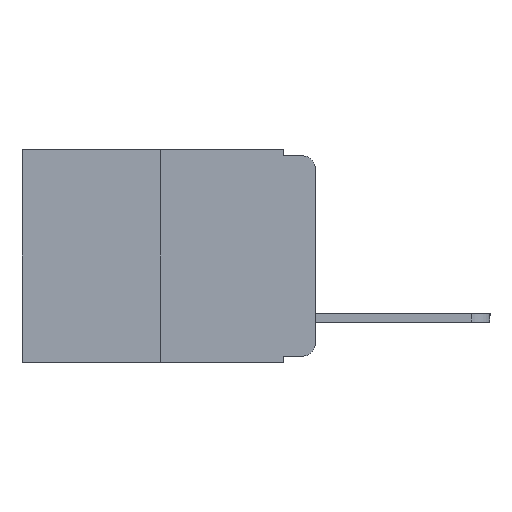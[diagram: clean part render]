
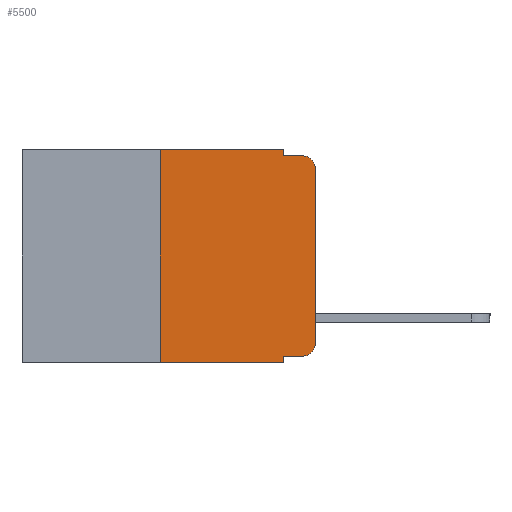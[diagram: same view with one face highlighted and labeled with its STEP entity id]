
A CAD part, left-side view. The second image highlights one B-rep face of the part: STEP entity #5500.
In plain terms, the highlighted planar face has unit normal (-1, 0, 0).
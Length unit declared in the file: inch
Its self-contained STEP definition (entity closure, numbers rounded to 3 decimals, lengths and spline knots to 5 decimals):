
#333 = VERTEX_POINT ( 'NONE', #11240 ) ;
#370 = LINE ( 'NONE', #1145, #9718 ) ;
#388 = CIRCLE ( 'NONE', #5598, 0.02 ) ;
#451 = VERTEX_POINT ( 'NONE', #4554 ) ;
#977 = DIRECTION ( 'NONE',  ( 0., -1., 0. ) ) ;
#1043 = DIRECTION ( 'NONE',  ( 0., -1., 0. ) ) ;
#1145 = CARTESIAN_POINT ( 'NONE',  ( 0., 0.473, 0. ) ) ;
#1429 = VERTEX_POINT ( 'NONE', #10984 ) ;
#1430 = VERTEX_POINT ( 'NONE', #10997 ) ;
#1515 = EDGE_CURVE ( 'NONE', #451, #1429, #10288, .T. ) ;
#1613 = CARTESIAN_POINT ( 'NONE',  ( 0., 0., 0. ) ) ;
#1649 = VERTEX_POINT ( 'NONE', #6279 ) ;
#1702 = DIRECTION ( 'NONE',  ( -1., 0., 0. ) ) ;
#1745 = CARTESIAN_POINT ( 'NONE',  ( 0., 0.051, -0.343 ) ) ;
#1945 = LINE ( 'NONE', #4502, #10922 ) ;
#2081 = VERTEX_POINT ( 'NONE', #5984 ) ;
#2215 = VECTOR ( 'NONE', #11425, 39.37008 ) ;
#2300 = CARTESIAN_POINT ( 'NONE',  ( 0., 0.473, -0.343 ) ) ;
#2356 = ORIENTED_EDGE ( 'NONE', *, *, #10770, .T. ) ;
#2634 = LINE ( 'NONE', #7529, #9096 ) ;
#2791 = ORIENTED_EDGE ( 'NONE', *, *, #8712, .F. ) ;
#3426 = DIRECTION ( 'NONE',  ( 0., 0., 1. ) ) ;
#3429 = VERTEX_POINT ( 'NONE', #6857 ) ;
#3449 = LINE ( 'NONE', #7114, #5597 ) ;
#4209 = EDGE_LOOP ( 'NONE', ( #5742, #10328, #10606, #4535, #4773, #2791, #10747, #4414, #11284, #2356 ) ) ;
#4414 = ORIENTED_EDGE ( 'NONE', *, *, #9178, .F. ) ;
#4502 = CARTESIAN_POINT ( 'NONE',  ( 0., 0.051, -0.01 ) ) ;
#4535 = ORIENTED_EDGE ( 'NONE', *, *, #8375, .F. ) ;
#4554 = CARTESIAN_POINT ( 'NONE',  ( 0., 0., -0.03 ) ) ;
#4773 = ORIENTED_EDGE ( 'NONE', *, *, #5081, .F. ) ;
#5035 = VERTEX_POINT ( 'NONE', #1745 ) ;
#5081 = EDGE_CURVE ( 'NONE', #3429, #333, #370, .T. ) ;
#5314 = LINE ( 'NONE', #1613, #2215 ) ;
#5500 = ADVANCED_FACE ( 'NONE', ( #10286 ), #10332, .F. ) ;
#5597 = VECTOR ( 'NONE', #3426, 39.37008 ) ;
#5598 = AXIS2_PLACEMENT_3D ( 'NONE', #7324, #1702, #8213 ) ;
#5742 = ORIENTED_EDGE ( 'NONE', *, *, #8959, .T. ) ;
#5748 = CARTESIAN_POINT ( 'NONE',  ( 0., 0.051, -0.333 ) ) ;
#5984 = CARTESIAN_POINT ( 'NONE',  ( 0., 0.02, -0.333 ) ) ;
#6279 = CARTESIAN_POINT ( 'NONE',  ( 0., 0., -0.313 ) ) ;
#6449 = VERTEX_POINT ( 'NONE', #8722 ) ;
#6453 = VECTOR ( 'NONE', #6993, 39.37008 ) ;
#6857 = CARTESIAN_POINT ( 'NONE',  ( 0., 0.25, 0. ) ) ;
#6993 = DIRECTION ( 'NONE',  ( 0., -1., 0. ) ) ;
#7114 = CARTESIAN_POINT ( 'NONE',  ( 0., 0.25, 0. ) ) ;
#7324 = CARTESIAN_POINT ( 'NONE',  ( 0., 0.02, -0.313 ) ) ;
#7333 = VERTEX_POINT ( 'NONE', #11731 ) ;
#7509 = CARTESIAN_POINT ( 'NONE',  ( 0., 0.051, 0. ) ) ;
#7529 = CARTESIAN_POINT ( 'NONE',  ( 0., 0.051, 0. ) ) ;
#7756 = EDGE_CURVE ( 'NONE', #1430, #1429, #1945, .T. ) ;
#8116 = DIRECTION ( 'NONE',  ( 0., -1., 0. ) ) ;
#8213 = DIRECTION ( 'NONE',  ( 0., 0., -1. ) ) ;
#8375 = EDGE_CURVE ( 'NONE', #333, #1430, #10234, .T. ) ;
#8395 = DIRECTION ( 'NONE',  ( 0., 0., -1. ) ) ;
#8614 = EDGE_CURVE ( 'NONE', #6449, #5035, #11290, .T. ) ;
#8712 = EDGE_CURVE ( 'NONE', #6449, #3429, #3449, .T. ) ;
#8722 = CARTESIAN_POINT ( 'NONE',  ( 0., 0.25, -0.343 ) ) ;
#8959 = EDGE_CURVE ( 'NONE', #1649, #451, #5314, .T. ) ;
#9096 = VECTOR ( 'NONE', #10054, 39.37008 ) ;
#9138 = CARTESIAN_POINT ( 'NONE',  ( 0., 0.473, 0. ) ) ;
#9178 = EDGE_CURVE ( 'NONE', #7333, #5035, #2634, .T. ) ;
#9224 = AXIS2_PLACEMENT_3D ( 'NONE', #9138, #10496, #10490 ) ;
#9230 = EDGE_CURVE ( 'NONE', #7333, #2081, #11019, .T. ) ;
#9594 = AXIS2_PLACEMENT_3D ( 'NONE', #10222, #10212, #10183 ) ;
#9718 = VECTOR ( 'NONE', #1043, 39.37008 ) ;
#10054 = DIRECTION ( 'NONE',  ( 0., 0., -1. ) ) ;
#10183 = DIRECTION ( 'NONE',  ( 0., 0., -1. ) ) ;
#10212 = DIRECTION ( 'NONE',  ( -1., 0., 0. ) ) ;
#10222 = CARTESIAN_POINT ( 'NONE',  ( 0., 0.02, -0.03 ) ) ;
#10234 = LINE ( 'NONE', #7509, #11633 ) ;
#10286 = FACE_OUTER_BOUND ( 'NONE', #4209, .T. ) ;
#10288 = CIRCLE ( 'NONE', #9594, 0.02 ) ;
#10328 = ORIENTED_EDGE ( 'NONE', *, *, #1515, .T. ) ;
#10332 = PLANE ( 'NONE',  #9224 ) ;
#10490 = DIRECTION ( 'NONE',  ( 0., 0., -1. ) ) ;
#10496 = DIRECTION ( 'NONE',  ( 1., 0., 0. ) ) ;
#10606 = ORIENTED_EDGE ( 'NONE', *, *, #7756, .F. ) ;
#10737 = VECTOR ( 'NONE', #977, 39.37008 ) ;
#10747 = ORIENTED_EDGE ( 'NONE', *, *, #8614, .T. ) ;
#10770 = EDGE_CURVE ( 'NONE', #2081, #1649, #388, .T. ) ;
#10922 = VECTOR ( 'NONE', #8116, 39.37008 ) ;
#10984 = CARTESIAN_POINT ( 'NONE',  ( 0., 0.02, -0.01 ) ) ;
#10997 = CARTESIAN_POINT ( 'NONE',  ( 0., 0.051, -0.01 ) ) ;
#11019 = LINE ( 'NONE', #5748, #10737 ) ;
#11240 = CARTESIAN_POINT ( 'NONE',  ( 0., 0.051, 0. ) ) ;
#11284 = ORIENTED_EDGE ( 'NONE', *, *, #9230, .T. ) ;
#11290 = LINE ( 'NONE', #2300, #6453 ) ;
#11425 = DIRECTION ( 'NONE',  ( 0., 0., 1. ) ) ;
#11633 = VECTOR ( 'NONE', #8395, 39.37008 ) ;
#11731 = CARTESIAN_POINT ( 'NONE',  ( 0., 0.051, -0.333 ) ) ;
